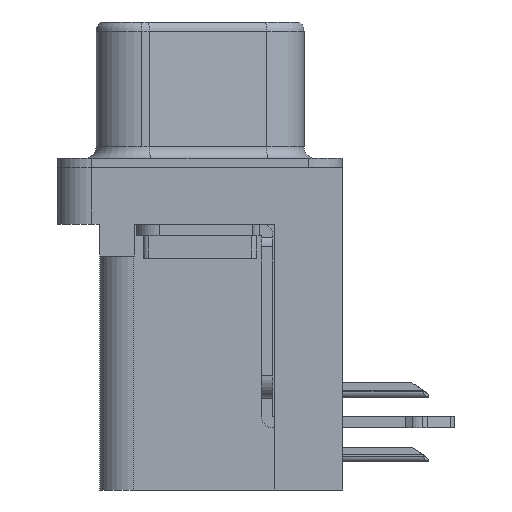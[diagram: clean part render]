
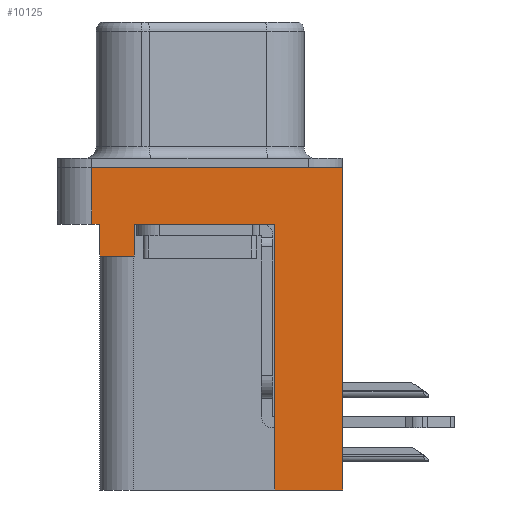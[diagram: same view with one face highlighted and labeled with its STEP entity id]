
A CAD part, left-side view. The second image highlights one B-rep face of the part: STEP entity #10125.
In plain terms, the highlighted planar face has unit normal (-1, 0, 0).
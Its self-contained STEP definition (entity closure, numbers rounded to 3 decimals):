
#363 = ORIENTED_EDGE ( 'NONE', *, *, #22458, .F. ) ;
#468 = VECTOR ( 'NONE', #19070, 1000. ) ;
#489 = ORIENTED_EDGE ( 'NONE', *, *, #13174, .T. ) ;
#596 = LINE ( 'NONE', #18738, #15183 ) ;
#681 = CARTESIAN_POINT ( 'NONE',  ( -3., -3.295, -14.2 ) ) ;
#982 = CARTESIAN_POINT ( 'NONE',  ( -3., -3.295, -14.2 ) ) ;
#1107 = VERTEX_POINT ( 'NONE', #982 ) ;
#1157 = ORIENTED_EDGE ( 'NONE', *, *, #17818, .F. ) ;
#1220 = VERTEX_POINT ( 'NONE', #8622 ) ;
#1703 = VECTOR ( 'NONE', #2569, 1000. ) ;
#1778 = EDGE_CURVE ( 'NONE', #7121, #21714, #10474, .T. ) ;
#1981 = DIRECTION ( 'NONE',  ( 0., 0., 1. ) ) ;
#2031 = VERTEX_POINT ( 'NONE', #22490 ) ;
#2311 = ORIENTED_EDGE ( 'NONE', *, *, #19122, .F. ) ;
#2555 = VERTEX_POINT ( 'NONE', #19124 ) ;
#2569 = DIRECTION ( 'NONE',  ( 0., 0., 1. ) ) ;
#2708 = VERTEX_POINT ( 'NONE', #17703 ) ;
#3990 = VECTOR ( 'NONE', #17164, 1000. ) ;
#4224 = CARTESIAN_POINT ( 'NONE',  ( -3., -6.275, -2.5 ) ) ;
#4716 = CARTESIAN_POINT ( 'NONE',  ( -3., 4.425, -3.9 ) ) ;
#4928 = CARTESIAN_POINT ( 'NONE',  ( -3., 4.775, -2.5 ) ) ;
#6097 = LINE ( 'NONE', #4224, #1703 ) ;
#6569 = CARTESIAN_POINT ( 'NONE',  ( -3., 2.895, -2.5 ) ) ;
#6696 = LINE ( 'NONE', #21424, #8606 ) ;
#6742 = DIRECTION ( 'NONE',  ( 0., 0., 1. ) ) ;
#6918 = LINE ( 'NONE', #4928, #14251 ) ;
#6932 = VECTOR ( 'NONE', #1981, 1000. ) ;
#7121 = VERTEX_POINT ( 'NONE', #15758 ) ;
#7882 = ORIENTED_EDGE ( 'NONE', *, *, #17019, .F. ) ;
#8248 = EDGE_LOOP ( 'NONE', ( #363, #21467, #489, #1157, #7882, #13809, #16031, #19707, #2311, #21388 ) ) ;
#8498 = PLANE ( 'NONE',  #16984 ) ;
#8606 = VECTOR ( 'NONE', #19412, 1000. ) ;
#8622 = CARTESIAN_POINT ( 'NONE',  ( -3., -6.275, 0. ) ) ;
#9641 = VECTOR ( 'NONE', #16889, 1000. ) ;
#10125 = ADVANCED_FACE ( 'NONE', ( #21234 ), #8498, .T. ) ;
#10474 = LINE ( 'NONE', #10704, #22872 ) ;
#10573 = VERTEX_POINT ( 'NONE', #4716 ) ;
#10605 = VERTEX_POINT ( 'NONE', #19322 ) ;
#10704 = CARTESIAN_POINT ( 'NONE',  ( -3., 2.895, -3.9 ) ) ;
#11340 = LINE ( 'NONE', #18304, #13413 ) ;
#11418 = DIRECTION ( 'NONE',  ( 0., -1., 0. ) ) ;
#11735 = LINE ( 'NONE', #20802, #3990 ) ;
#12825 = LINE ( 'NONE', #681, #6932 ) ;
#13174 = EDGE_CURVE ( 'NONE', #17336, #10605, #20947, .T. ) ;
#13413 = VECTOR ( 'NONE', #20067, 1000. ) ;
#13542 = CARTESIAN_POINT ( 'NONE',  ( -3., -6.275, -2.5 ) ) ;
#13809 = ORIENTED_EDGE ( 'NONE', *, *, #1778, .T. ) ;
#14146 = DIRECTION ( 'NONE',  ( 0., 0., 1. ) ) ;
#14251 = VECTOR ( 'NONE', #15991, 1000. ) ;
#14391 = EDGE_CURVE ( 'NONE', #21714, #2555, #596, .T. ) ;
#15183 = VECTOR ( 'NONE', #11418, 1000. ) ;
#15404 = EDGE_CURVE ( 'NONE', #1107, #2555, #12825, .T. ) ;
#15700 = CARTESIAN_POINT ( 'NONE',  ( -3., -6.275, -2.5 ) ) ;
#15758 = CARTESIAN_POINT ( 'NONE',  ( -3., 2.895, -3.9 ) ) ;
#15991 = DIRECTION ( 'NONE',  ( 0., 0., 1. ) ) ;
#16031 = ORIENTED_EDGE ( 'NONE', *, *, #14391, .T. ) ;
#16675 = CARTESIAN_POINT ( 'NONE',  ( -3., 4.775, -2.5 ) ) ;
#16844 = EDGE_CURVE ( 'NONE', #2708, #1220, #6097, .T. ) ;
#16889 = DIRECTION ( 'NONE',  ( 0., 1., 0. ) ) ;
#16984 = AXIS2_PLACEMENT_3D ( 'NONE', #15700, #22890, #6742 ) ;
#17019 = EDGE_CURVE ( 'NONE', #7121, #10573, #11735, .T. ) ;
#17164 = DIRECTION ( 'NONE',  ( 0., 1., 0. ) ) ;
#17336 = VERTEX_POINT ( 'NONE', #16675 ) ;
#17703 = CARTESIAN_POINT ( 'NONE',  ( -3., -6.275, -14.2 ) ) ;
#17818 = EDGE_CURVE ( 'NONE', #10573, #10605, #11340, .T. ) ;
#18304 = CARTESIAN_POINT ( 'NONE',  ( -3., 4.425, -3.9 ) ) ;
#18738 = CARTESIAN_POINT ( 'NONE',  ( -3., -6.275, -2.5 ) ) ;
#19070 = DIRECTION ( 'NONE',  ( 0., -1., 0. ) ) ;
#19122 = EDGE_CURVE ( 'NONE', #2708, #1107, #22319, .T. ) ;
#19124 = CARTESIAN_POINT ( 'NONE',  ( -3., -3.295, -2.5 ) ) ;
#19322 = CARTESIAN_POINT ( 'NONE',  ( -3., 4.425, -2.5 ) ) ;
#19412 = DIRECTION ( 'NONE',  ( 0., -1., 0. ) ) ;
#19707 = ORIENTED_EDGE ( 'NONE', *, *, #15404, .F. ) ;
#20067 = DIRECTION ( 'NONE',  ( 0., 0., 1. ) ) ;
#20753 = CARTESIAN_POINT ( 'NONE',  ( -3., -3.295, -14.2 ) ) ;
#20802 = CARTESIAN_POINT ( 'NONE',  ( -3., 4.425, -3.9 ) ) ;
#20947 = LINE ( 'NONE', #13542, #468 ) ;
#21234 = FACE_OUTER_BOUND ( 'NONE', #8248, .T. ) ;
#21388 = ORIENTED_EDGE ( 'NONE', *, *, #16844, .T. ) ;
#21424 = CARTESIAN_POINT ( 'NONE',  ( -3., -6.275, 0. ) ) ;
#21467 = ORIENTED_EDGE ( 'NONE', *, *, #21773, .F. ) ;
#21714 = VERTEX_POINT ( 'NONE', #6569 ) ;
#21773 = EDGE_CURVE ( 'NONE', #17336, #2031, #6918, .T. ) ;
#22319 = LINE ( 'NONE', #20753, #9641 ) ;
#22458 = EDGE_CURVE ( 'NONE', #2031, #1220, #6696, .T. ) ;
#22490 = CARTESIAN_POINT ( 'NONE',  ( -3., 4.775, 0. ) ) ;
#22872 = VECTOR ( 'NONE', #14146, 1000. ) ;
#22890 = DIRECTION ( 'NONE',  ( -1., 0., 0. ) ) ;
